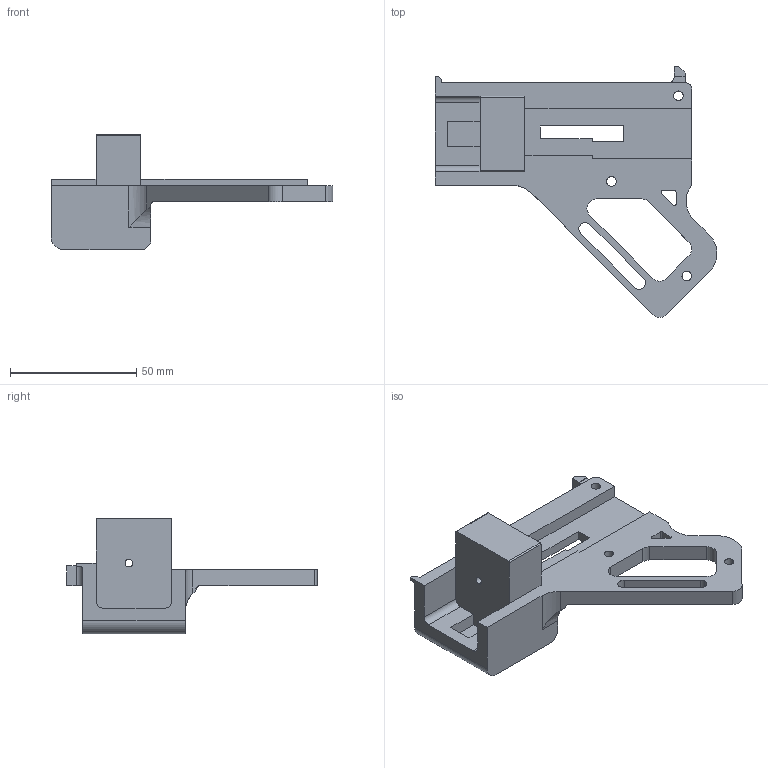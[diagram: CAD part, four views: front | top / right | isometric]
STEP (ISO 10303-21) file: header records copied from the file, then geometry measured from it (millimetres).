
FILE_DESCRIPTION (( 'STEP AP214' ), '1' );
FILE_NAME ('frame_l.STEP', '2014-01-22T21:34:22', ( '' ), ( '' ), 'SwSTEP 2.0', 'SolidWorks 2013', '' );
FILE_SCHEMA (( 'AUTOMOTIVE_DESIGN' ));
Length unit declared in the file: inch
Products named in the file (1): frame_l
Bounding box: 111.61 x 99.3 x 45.72 mm (x, y, z)
Volume: 64009.8 mm3; surface area: 21344.9 mm2
Topology: 1 solids, 1 shells, 163 faces, 450 edges, 295 vertices
Faces by surface type: plane 96, cylinder 43, bspline 21, torus 2, sphere 1
Entity records: 6374 total; most frequent: CARTESIAN_POINT 2235, ORIENTED_EDGE 898, DIRECTION 768, EDGE_CURVE 449, VECTOR 320, LINE 320, VERTEX_POINT 295, AXIS2_PLACEMENT_3D 224
